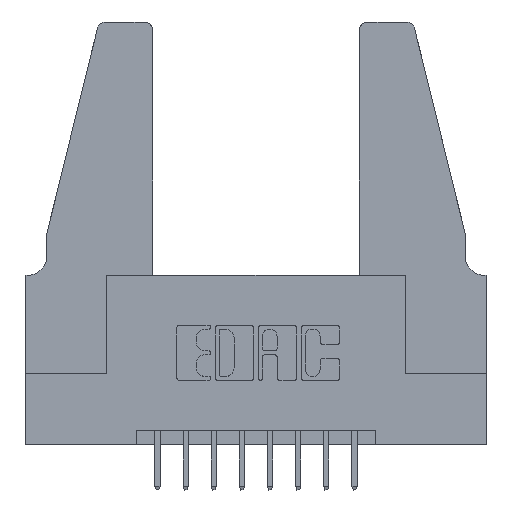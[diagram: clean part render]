
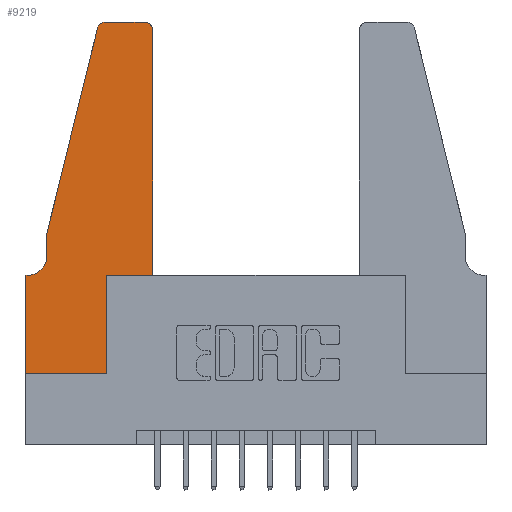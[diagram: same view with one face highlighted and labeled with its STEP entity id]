
A CAD part, top view. The second image highlights one B-rep face of the part: STEP entity #9219.
In plain terms, the highlighted planar face has unit normal (0, 0, 1).
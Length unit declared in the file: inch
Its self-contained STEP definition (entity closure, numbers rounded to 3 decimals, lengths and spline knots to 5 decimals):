
#4 = EDGE_CURVE ( 'NONE', #8388, #5590, #6114, .T. ) ;
#71 = CIRCLE ( 'NONE', #10337, 0.03 ) ;
#159 = ORIENTED_EDGE ( 'NONE', *, *, #10492, .T. ) ;
#336 = CARTESIAN_POINT ( 'NONE',  ( 0., 0.35, 0.37 ) ) ;
#382 = VECTOR ( 'NONE', #7049, 39.37008 ) ;
#442 = FACE_OUTER_BOUND ( 'NONE', #6688, .T. ) ;
#445 = CARTESIAN_POINT ( 'NONE',  ( 0., 0.35, 0.37 ) ) ;
#477 = CARTESIAN_POINT ( 'NONE',  ( 0.0055, 0.42, 0.37 ) ) ;
#490 = ORIENTED_EDGE ( 'NONE', *, *, #11309, .T. ) ;
#532 = ORIENTED_EDGE ( 'NONE', *, *, #12146, .T. ) ;
#533 = LINE ( 'NONE', #2226, #5681 ) ;
#826 = DIRECTION ( 'NONE',  ( 0., 0., 1. ) ) ;
#984 = EDGE_CURVE ( 'NONE', #1261, #7911, #10174, .T. ) ;
#1261 = VERTEX_POINT ( 'NONE', #2381 ) ;
#1324 = LINE ( 'NONE', #1380, #1641 ) ;
#1332 = CARTESIAN_POINT ( 'NONE',  ( 0.284, 1.22, 0.37 ) ) ;
#1344 = CARTESIAN_POINT ( 'NONE',  ( 0.2865, 0.35, 0.37 ) ) ;
#1348 = DIRECTION ( 'NONE',  ( 1., 0., 0. ) ) ;
#1380 = CARTESIAN_POINT ( 'NONE',  ( 0.0755, 0.35, 0.37 ) ) ;
#1481 = VECTOR ( 'NONE', #6157, 39.37008 ) ;
#1486 = DIRECTION ( 'NONE',  ( -1., 0., 0. ) ) ;
#1641 = VECTOR ( 'NONE', #8553, 39.37008 ) ;
#2158 = VERTEX_POINT ( 'NONE', #1344 ) ;
#2226 = CARTESIAN_POINT ( 'NONE',  ( 0.0755, 0.5, 0.37 ) ) ;
#2378 = DIRECTION ( 'NONE',  ( 1., 0., 0. ) ) ;
#2381 = CARTESIAN_POINT ( 'NONE',  ( 0.0755, 0.5, 0.37 ) ) ;
#2480 = VECTOR ( 'NONE', #11385, 39.37008 ) ;
#2527 = AXIS2_PLACEMENT_3D ( 'NONE', #477, #7636, #1486 ) ;
#2563 = DIRECTION ( 'NONE',  ( 1., 0., 0. ) ) ;
#2630 = LINE ( 'NONE', #5354, #2480 ) ;
#2903 = CARTESIAN_POINT ( 'NONE',  ( 0.25487, 1.22718, 0.37 ) ) ;
#3168 = AXIS2_PLACEMENT_3D ( 'NONE', #1332, #8509, #2378 ) ;
#3372 = VECTOR ( 'NONE', #11059, 39.37008 ) ;
#3483 = VECTOR ( 'NONE', #2563, 39.37008 ) ;
#3488 = ORIENTED_EDGE ( 'NONE', *, *, #12169, .T. ) ;
#3527 = ORIENTED_EDGE ( 'NONE', *, *, #12514, .T. ) ;
#3590 = CARTESIAN_POINT ( 'NONE',  ( 0., 0., 0.37 ) ) ;
#4042 = CARTESIAN_POINT ( 'NONE',  ( 0.2605, 1.25, 0.37 ) ) ;
#4206 = CARTESIAN_POINT ( 'NONE',  ( 0., 0., 0.37 ) ) ;
#4507 = CARTESIAN_POINT ( 'NONE',  ( 0.284, 1.25, 0.37 ) ) ;
#4792 = VECTOR ( 'NONE', #10396, 39.37008 ) ;
#4818 = ORIENTED_EDGE ( 'NONE', *, *, #8776, .T. ) ;
#5300 = EDGE_CURVE ( 'NONE', #5590, #12511, #71, .T. ) ;
#5354 = CARTESIAN_POINT ( 'NONE',  ( 0., 0., 0.37 ) ) ;
#5536 = LINE ( 'NONE', #9199, #1481 ) ;
#5590 = VERTEX_POINT ( 'NONE', #11345 ) ;
#5681 = VECTOR ( 'NONE', #8310, 39.37008 ) ;
#5703 = EDGE_CURVE ( 'NONE', #5794, #10462, #1324, .T. ) ;
#5794 = VERTEX_POINT ( 'NONE', #9687 ) ;
#6025 = CARTESIAN_POINT ( 'NONE',  ( 0.4505, 0.35, 0.37 ) ) ;
#6114 = LINE ( 'NONE', #9061, #3372 ) ;
#6157 = DIRECTION ( 'NONE',  ( 0., 1., 0. ) ) ;
#6347 = CARTESIAN_POINT ( 'NONE',  ( 0.0755, 0.42, 0.37 ) ) ;
#6366 = ORIENTED_EDGE ( 'NONE', *, *, #4, .T. ) ;
#6688 = EDGE_LOOP ( 'NONE', ( #490, #3488, #11968, #7554, #4818, #12005, #532, #159, #9924, #3527, #6366, #12887 ) ) ;
#6977 = CARTESIAN_POINT ( 'NONE',  ( 0.4205, 1.22, 0.37 ) ) ;
#7049 = DIRECTION ( 'NONE',  ( 1., 0., 0. ) ) ;
#7494 = DIRECTION ( 'NONE',  ( 0., 0., 1. ) ) ;
#7554 = ORIENTED_EDGE ( 'NONE', *, *, #984, .T. ) ;
#7636 = DIRECTION ( 'NONE',  ( 0., 0., -1. ) ) ;
#7846 = VERTEX_POINT ( 'NONE', #4206 ) ;
#7911 = VERTEX_POINT ( 'NONE', #6347 ) ;
#7972 = DIRECTION ( 'NONE',  ( 1., 0., 0. ) ) ;
#8310 = DIRECTION ( 'NONE',  ( -0.239, -0.971, 0. ) ) ;
#8388 = VERTEX_POINT ( 'NONE', #12052 ) ;
#8509 = DIRECTION ( 'NONE',  ( 0., 0., 1. ) ) ;
#8544 = LINE ( 'NONE', #6025, #382 ) ;
#8545 = CARTESIAN_POINT ( 'NONE',  ( 0.2865, 0., 0.37 ) ) ;
#8553 = DIRECTION ( 'NONE',  ( -1., 0., 0. ) ) ;
#8776 = EDGE_CURVE ( 'NONE', #7911, #5794, #11265, .T. ) ;
#8901 = LINE ( 'NONE', #3590, #3483 ) ;
#9020 = CARTESIAN_POINT ( 'NONE',  ( 0.4205, 1.25, 0.37 ) ) ;
#9061 = CARTESIAN_POINT ( 'NONE',  ( 0.4505, 0.35, 0.37 ) ) ;
#9199 = CARTESIAN_POINT ( 'NONE',  ( 0.2865, 0.35, 0.37 ) ) ;
#9219 = ADVANCED_FACE ( 'NONE', ( #442 ), #10484, .T. ) ;
#9687 = CARTESIAN_POINT ( 'NONE',  ( 0.0055, 0.35, 0.37 ) ) ;
#9924 = ORIENTED_EDGE ( 'NONE', *, *, #12656, .T. ) ;
#9951 = VERTEX_POINT ( 'NONE', #4507 ) ;
#10174 = LINE ( 'NONE', #10280, #4792 ) ;
#10280 = CARTESIAN_POINT ( 'NONE',  ( 0.0755, 0.5, 0.37 ) ) ;
#10337 = AXIS2_PLACEMENT_3D ( 'NONE', #6977, #826, #7972 ) ;
#10396 = DIRECTION ( 'NONE',  ( 0., -1., 0. ) ) ;
#10462 = VERTEX_POINT ( 'NONE', #445 ) ;
#10484 = PLANE ( 'NONE',  #11125 ) ;
#10492 = EDGE_CURVE ( 'NONE', #7846, #12226, #8901, .T. ) ;
#11059 = DIRECTION ( 'NONE',  ( 0., 1., 0. ) ) ;
#11104 = DIRECTION ( 'NONE',  ( -1., 0., 0. ) ) ;
#11125 = AXIS2_PLACEMENT_3D ( 'NONE', #336, #7494, #1348 ) ;
#11265 = CIRCLE ( 'NONE', #2527, 0.07 ) ;
#11309 = EDGE_CURVE ( 'NONE', #12511, #9951, #12425, .T. ) ;
#11345 = CARTESIAN_POINT ( 'NONE',  ( 0.4505, 1.22, 0.37 ) ) ;
#11385 = DIRECTION ( 'NONE',  ( 0., -1., 0. ) ) ;
#11924 = VERTEX_POINT ( 'NONE', #2903 ) ;
#11968 = ORIENTED_EDGE ( 'NONE', *, *, #12752, .T. ) ;
#12005 = ORIENTED_EDGE ( 'NONE', *, *, #5703, .T. ) ;
#12052 = CARTESIAN_POINT ( 'NONE',  ( 0.4505, 0.35, 0.37 ) ) ;
#12146 = EDGE_CURVE ( 'NONE', #10462, #7846, #2630, .T. ) ;
#12169 = EDGE_CURVE ( 'NONE', #9951, #11924, #12895, .T. ) ;
#12226 = VERTEX_POINT ( 'NONE', #8545 ) ;
#12425 = LINE ( 'NONE', #4042, #12746 ) ;
#12511 = VERTEX_POINT ( 'NONE', #9020 ) ;
#12514 = EDGE_CURVE ( 'NONE', #2158, #8388, #8544, .T. ) ;
#12656 = EDGE_CURVE ( 'NONE', #12226, #2158, #5536, .T. ) ;
#12746 = VECTOR ( 'NONE', #11104, 39.37008 ) ;
#12752 = EDGE_CURVE ( 'NONE', #11924, #1261, #533, .T. ) ;
#12887 = ORIENTED_EDGE ( 'NONE', *, *, #5300, .T. ) ;
#12895 = CIRCLE ( 'NONE', #3168, 0.03 ) ;
